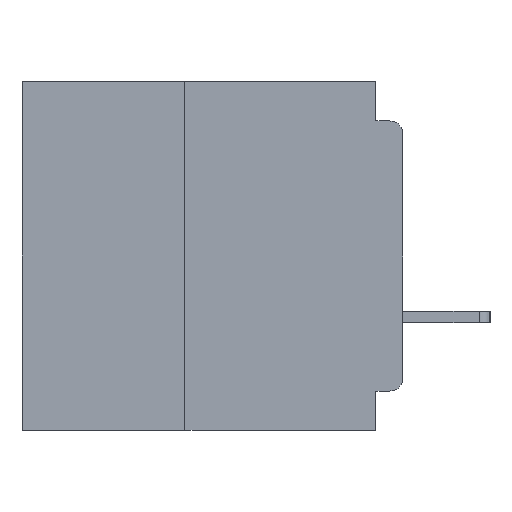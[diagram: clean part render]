
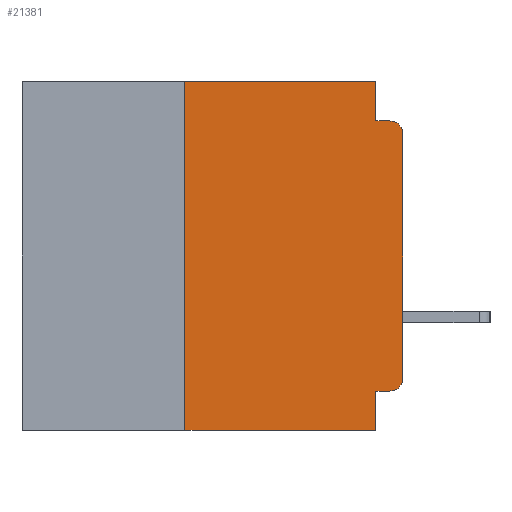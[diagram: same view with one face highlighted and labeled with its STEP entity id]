
A CAD part, left-side view. The second image highlights one B-rep face of the part: STEP entity #21381.
In plain terms, the highlighted planar face has unit normal (-1, 0, 0).
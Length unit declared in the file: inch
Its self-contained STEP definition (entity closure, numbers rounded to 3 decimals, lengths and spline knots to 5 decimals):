
#157 = DIRECTION ( 'NONE',  ( 0., 1., 0. ) ) ;
#1266 = VECTOR ( 'NONE', #24155, 39.37008 ) ;
#2205 = CARTESIAN_POINT ( 'NONE',  ( 0., 0.437, 0. ) ) ;
#2633 = LINE ( 'NONE', #15778, #1266 ) ;
#2753 = VERTEX_POINT ( 'NONE', #26155 ) ;
#2914 = DIRECTION ( 'NONE',  ( -1., 0., 0. ) ) ;
#3027 = LINE ( 'NONE', #32536, #37139 ) ;
#3061 = ORIENTED_EDGE ( 'NONE', *, *, #13385, .T. ) ;
#3405 = VECTOR ( 'NONE', #26560, 39.37008 ) ;
#4030 = AXIS2_PLACEMENT_3D ( 'NONE', #2205, #41642, #16245 ) ;
#4643 = ORIENTED_EDGE ( 'NONE', *, *, #41768, .T. ) ;
#5400 = ORIENTED_EDGE ( 'NONE', *, *, #12027, .T. ) ;
#6417 = VERTEX_POINT ( 'NONE', #23864 ) ;
#8116 = CARTESIAN_POINT ( 'NONE',  ( 0., 0.031, -0.4 ) ) ;
#8882 = AXIS2_PLACEMENT_3D ( 'NONE', #28596, #2914, #32865 ) ;
#9343 = VECTOR ( 'NONE', #17052, 39.37008 ) ;
#10026 = VECTOR ( 'NONE', #157, 39.37008 ) ;
#10514 = CIRCLE ( 'NONE', #8882, 0.015 ) ;
#10680 = CARTESIAN_POINT ( 'NONE',  ( 0., 0.031, 0. ) ) ;
#11623 = VERTEX_POINT ( 'NONE', #10680 ) ;
#12027 = EDGE_CURVE ( 'NONE', #16927, #13320, #48650, .T. ) ;
#12183 = ORIENTED_EDGE ( 'NONE', *, *, #39147, .T. ) ;
#13320 = VERTEX_POINT ( 'NONE', #43278 ) ;
#13385 = EDGE_CURVE ( 'NONE', #42962, #6417, #39209, .T. ) ;
#13765 = VERTEX_POINT ( 'NONE', #46325 ) ;
#13796 = VECTOR ( 'NONE', #23500, 39.37008 ) ;
#14478 = DIRECTION ( 'NONE',  ( 0., 0., 1. ) ) ;
#15359 = EDGE_CURVE ( 'NONE', #11623, #36298, #37741, .T. ) ;
#15778 = CARTESIAN_POINT ( 'NONE',  ( 0., 0., -0.045 ) ) ;
#16167 = ORIENTED_EDGE ( 'NONE', *, *, #46020, .F. ) ;
#16245 = DIRECTION ( 'NONE',  ( 0., 0., -1. ) ) ;
#16354 = LINE ( 'NONE', #39927, #38912 ) ;
#16927 = VERTEX_POINT ( 'NONE', #29456 ) ;
#17031 = ORIENTED_EDGE ( 'NONE', *, *, #30691, .F. ) ;
#17052 = DIRECTION ( 'NONE',  ( 0., 0., -1. ) ) ;
#17837 = CARTESIAN_POINT ( 'NONE',  ( 0., 0.015, -0.355 ) ) ;
#18429 = CARTESIAN_POINT ( 'NONE',  ( 0., 0.015, -0.06 ) ) ;
#19190 = CARTESIAN_POINT ( 'NONE',  ( 0., 0.031, 0. ) ) ;
#19554 = CARTESIAN_POINT ( 'NONE',  ( 0., 0., -0.06 ) ) ;
#20240 = ORIENTED_EDGE ( 'NONE', *, *, #15359, .F. ) ;
#20827 = LINE ( 'NONE', #8116, #9343 ) ;
#21381 = ADVANCED_FACE ( 'NONE', ( #50643 ), #53322, .F. ) ;
#21674 = VERTEX_POINT ( 'NONE', #52018 ) ;
#22215 = VERTEX_POINT ( 'NONE', #17837 ) ;
#22736 = DIRECTION ( 'NONE',  ( 0., 0., -1. ) ) ;
#23392 = CARTESIAN_POINT ( 'NONE',  ( 0., 0.25, -0.4 ) ) ;
#23500 = DIRECTION ( 'NONE',  ( 0., 0., -1. ) ) ;
#23864 = CARTESIAN_POINT ( 'NONE',  ( 0., 0.015, -0.045 ) ) ;
#24155 = DIRECTION ( 'NONE',  ( 0., -1., 0. ) ) ;
#25365 = AXIS2_PLACEMENT_3D ( 'NONE', #18429, #47987, #22736 ) ;
#26155 = CARTESIAN_POINT ( 'NONE',  ( 0., 0.031, -0.355 ) ) ;
#26560 = DIRECTION ( 'NONE',  ( 0., -1., 0. ) ) ;
#27647 = DIRECTION ( 'NONE',  ( 0., 0., 1. ) ) ;
#28155 = LINE ( 'NONE', #23392, #49246 ) ;
#28596 = CARTESIAN_POINT ( 'NONE',  ( 0., 0.015, -0.34 ) ) ;
#29456 = CARTESIAN_POINT ( 'NONE',  ( 0., 0.25, -0.4 ) ) ;
#29854 = EDGE_CURVE ( 'NONE', #36298, #6417, #2633, .T. ) ;
#30691 = EDGE_CURVE ( 'NONE', #22215, #2753, #44582, .T. ) ;
#32536 = CARTESIAN_POINT ( 'NONE',  ( 0., 0.437, 0. ) ) ;
#32865 = DIRECTION ( 'NONE',  ( 0., 0., -1. ) ) ;
#36267 = CARTESIAN_POINT ( 'NONE',  ( 0., 0.031, -0.045 ) ) ;
#36298 = VERTEX_POINT ( 'NONE', #36267 ) ;
#36815 = DIRECTION ( 'NONE',  ( 0., -1., 0. ) ) ;
#37139 = VECTOR ( 'NONE', #36815, 39.37008 ) ;
#37741 = LINE ( 'NONE', #19190, #13796 ) ;
#38517 = CARTESIAN_POINT ( 'NONE',  ( 0., 0., -0.355 ) ) ;
#38773 = CARTESIAN_POINT ( 'NONE',  ( 0., 0.437, -0.4 ) ) ;
#38912 = VECTOR ( 'NONE', #14478, 39.37008 ) ;
#39147 = EDGE_CURVE ( 'NONE', #21674, #42962, #16354, .T. ) ;
#39209 = CIRCLE ( 'NONE', #25365, 0.015 ) ;
#39927 = CARTESIAN_POINT ( 'NONE',  ( 0., 0., 0. ) ) ;
#41642 = DIRECTION ( 'NONE',  ( 1., 0., 0. ) ) ;
#41768 = EDGE_CURVE ( 'NONE', #22215, #21674, #10514, .T. ) ;
#42962 = VERTEX_POINT ( 'NONE', #19554 ) ;
#43278 = CARTESIAN_POINT ( 'NONE',  ( 0., 0.031, -0.4 ) ) ;
#44582 = LINE ( 'NONE', #38517, #10026 ) ;
#45231 = EDGE_LOOP ( 'NONE', ( #12183, #3061, #53033, #20240, #47009, #16167, #5400, #54602, #17031, #4643 ) ) ;
#46020 = EDGE_CURVE ( 'NONE', #16927, #13765, #28155, .T. ) ;
#46325 = CARTESIAN_POINT ( 'NONE',  ( 0., 0.25, 0. ) ) ;
#46344 = EDGE_CURVE ( 'NONE', #2753, #13320, #20827, .T. ) ;
#47009 = ORIENTED_EDGE ( 'NONE', *, *, #53174, .F. ) ;
#47987 = DIRECTION ( 'NONE',  ( -1., 0., 0. ) ) ;
#48650 = LINE ( 'NONE', #38773, #3405 ) ;
#49246 = VECTOR ( 'NONE', #27647, 39.37008 ) ;
#50643 = FACE_OUTER_BOUND ( 'NONE', #45231, .T. ) ;
#52018 = CARTESIAN_POINT ( 'NONE',  ( 0., 0., -0.34 ) ) ;
#53033 = ORIENTED_EDGE ( 'NONE', *, *, #29854, .F. ) ;
#53174 = EDGE_CURVE ( 'NONE', #13765, #11623, #3027, .T. ) ;
#53322 = PLANE ( 'NONE',  #4030 ) ;
#54602 = ORIENTED_EDGE ( 'NONE', *, *, #46344, .F. ) ;
